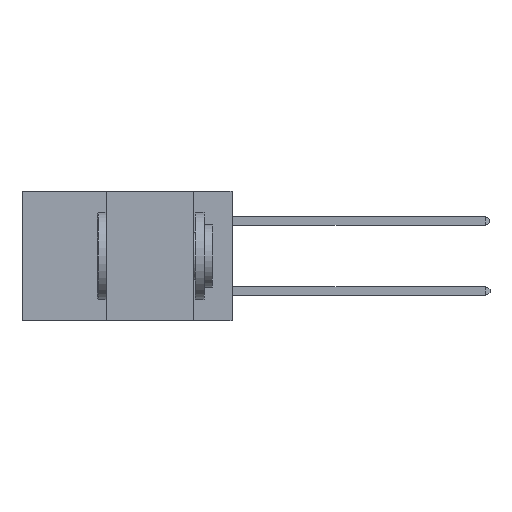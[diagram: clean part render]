
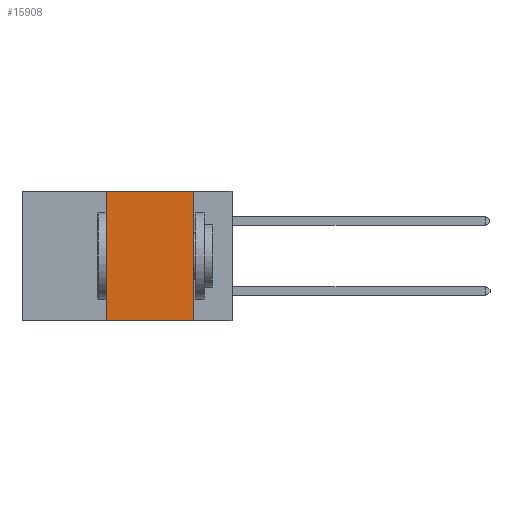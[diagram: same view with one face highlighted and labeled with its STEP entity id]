
A CAD part, left-side view. The second image highlights one B-rep face of the part: STEP entity #15908.
In plain terms, the highlighted planar face has unit normal (-1, 0, 0).
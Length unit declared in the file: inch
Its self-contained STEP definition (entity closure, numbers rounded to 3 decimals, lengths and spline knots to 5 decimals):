
#1547 = ORIENTED_EDGE ( 'NONE', *, *, #16109, .T. ) ;
#1655 = FACE_OUTER_BOUND ( 'NONE', #10981, .T. ) ;
#1856 = CARTESIAN_POINT ( 'NONE',  ( 0., 0.6, 0. ) ) ;
#1895 = VECTOR ( 'NONE', #5749, 39.37008 ) ;
#1980 = CARTESIAN_POINT ( 'NONE',  ( 0., 0.36, 0. ) ) ;
#2533 = VECTOR ( 'NONE', #4713, 39.37008 ) ;
#3547 = DIRECTION ( 'NONE',  ( 0., 0., -1. ) ) ;
#4357 = CARTESIAN_POINT ( 'NONE',  ( 0., 0.11, 0. ) ) ;
#4713 = DIRECTION ( 'NONE',  ( 0., -1., 0. ) ) ;
#5200 = VECTOR ( 'NONE', #17759, 39.37008 ) ;
#5279 = LINE ( 'NONE', #1980, #12621 ) ;
#5646 = LINE ( 'NONE', #4357, #1895 ) ;
#5749 = DIRECTION ( 'NONE',  ( 0., 0., -1. ) ) ;
#6260 = LINE ( 'NONE', #1856, #2533 ) ;
#6429 = CARTESIAN_POINT ( 'NONE',  ( 0., 0.36, 0. ) ) ;
#7519 = DIRECTION ( 'NONE',  ( 0., 0., 1. ) ) ;
#8862 = LINE ( 'NONE', #10875, #5200 ) ;
#9069 = PLANE ( 'NONE',  #13653 ) ;
#10875 = CARTESIAN_POINT ( 'NONE',  ( 0., 0.6, -0.37 ) ) ;
#10981 = EDGE_LOOP ( 'NONE', ( #11435, #12715, #13879, #1547 ) ) ;
#11435 = ORIENTED_EDGE ( 'NONE', *, *, #15661, .F. ) ;
#11845 = DIRECTION ( 'NONE',  ( 1., 0., 0. ) ) ;
#12081 = CARTESIAN_POINT ( 'NONE',  ( 0., 0.36, -0.37 ) ) ;
#12621 = VECTOR ( 'NONE', #7519, 39.37008 ) ;
#12715 = ORIENTED_EDGE ( 'NONE', *, *, #16296, .F. ) ;
#12930 = VERTEX_POINT ( 'NONE', #6429 ) ;
#13653 = AXIS2_PLACEMENT_3D ( 'NONE', #15938, #11845, #3547 ) ;
#13879 = ORIENTED_EDGE ( 'NONE', *, *, #13932, .F. ) ;
#13932 = EDGE_CURVE ( 'NONE', #14126, #12930, #5279, .T. ) ;
#14126 = VERTEX_POINT ( 'NONE', #12081 ) ;
#14297 = VERTEX_POINT ( 'NONE', #15194 ) ;
#14880 = VERTEX_POINT ( 'NONE', #17734 ) ;
#15194 = CARTESIAN_POINT ( 'NONE',  ( 0., 0.11, -0.37 ) ) ;
#15661 = EDGE_CURVE ( 'NONE', #14880, #14297, #5646, .T. ) ;
#15908 = ADVANCED_FACE ( 'NONE', ( #1655 ), #9069, .F. ) ;
#15938 = CARTESIAN_POINT ( 'NONE',  ( 0., 0.6, 0. ) ) ;
#16109 = EDGE_CURVE ( 'NONE', #14126, #14297, #8862, .T. ) ;
#16296 = EDGE_CURVE ( 'NONE', #12930, #14880, #6260, .T. ) ;
#17734 = CARTESIAN_POINT ( 'NONE',  ( 0., 0.11, 0. ) ) ;
#17759 = DIRECTION ( 'NONE',  ( 0., -1., 0. ) ) ;
